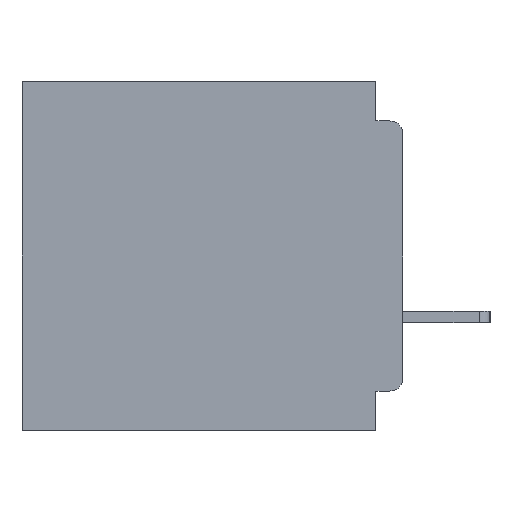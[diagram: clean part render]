
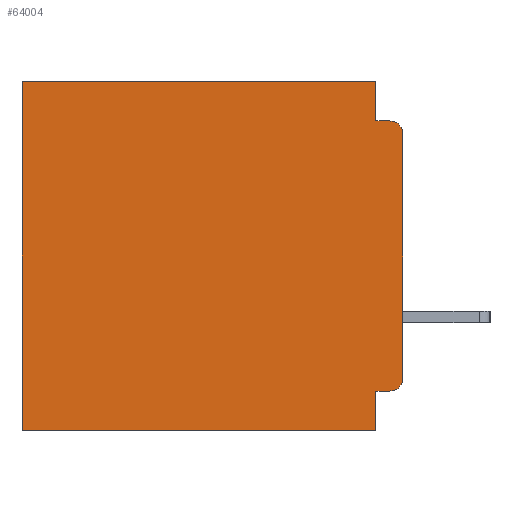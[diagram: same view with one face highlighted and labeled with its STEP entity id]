
A CAD part, left-side view. The second image highlights one B-rep face of the part: STEP entity #64004.
In plain terms, the highlighted planar face has unit normal (-1, 0, 0).
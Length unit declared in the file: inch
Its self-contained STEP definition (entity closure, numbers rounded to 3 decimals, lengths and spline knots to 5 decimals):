
#859 = CARTESIAN_POINT ( 'NONE',  ( 0.3, 0., -0.045 ) ) ;
#1046 = DIRECTION ( 'NONE',  ( 0., 0., -1. ) ) ;
#2041 = VERTEX_POINT ( 'NONE', #41027 ) ;
#2657 = VECTOR ( 'NONE', #32019, 39.37008 ) ;
#2817 = CIRCLE ( 'NONE', #4854, 0.015 ) ;
#3303 = VECTOR ( 'NONE', #16511, 39.37008 ) ;
#4626 = EDGE_LOOP ( 'NONE', ( #4662, #31064, #33483, #18555, #24308, #18602, #51033, #5411, #11930, #7686 ) ) ;
#4662 = ORIENTED_EDGE ( 'NONE', *, *, #42477, .F. ) ;
#4854 = AXIS2_PLACEMENT_3D ( 'NONE', #28053, #64151, #33227 ) ;
#5411 = ORIENTED_EDGE ( 'NONE', *, *, #32734, .F. ) ;
#6236 = CARTESIAN_POINT ( 'NONE',  ( 0.3, 0.437, -0.4 ) ) ;
#6506 = VECTOR ( 'NONE', #57713, 39.37008 ) ;
#6754 = CARTESIAN_POINT ( 'NONE',  ( 0.3, 0., -0.4 ) ) ;
#7686 = ORIENTED_EDGE ( 'NONE', *, *, #48527, .T. ) ;
#8101 = CARTESIAN_POINT ( 'NONE',  ( 0.3, 0., -0.06 ) ) ;
#9008 = EDGE_CURVE ( 'NONE', #2041, #52479, #17122, .T. ) ;
#9335 = CARTESIAN_POINT ( 'NONE',  ( 0.3, 0.031, 0. ) ) ;
#11239 = VECTOR ( 'NONE', #45523, 39.37008 ) ;
#11930 = ORIENTED_EDGE ( 'NONE', *, *, #64659, .F. ) ;
#12220 = DIRECTION ( 'NONE',  ( 0., 0., -1. ) ) ;
#13569 = DIRECTION ( 'NONE',  ( 0., 1., 0. ) ) ;
#13674 = CARTESIAN_POINT ( 'NONE',  ( 0.3, 0., -0.355 ) ) ;
#15152 = VECTOR ( 'NONE', #1046, 39.37008 ) ;
#15683 = VERTEX_POINT ( 'NONE', #22518 ) ;
#16511 = DIRECTION ( 'NONE',  ( 0., -1., 0. ) ) ;
#17122 = LINE ( 'NONE', #859, #3303 ) ;
#18555 = ORIENTED_EDGE ( 'NONE', *, *, #24389, .F. ) ;
#18602 = ORIENTED_EDGE ( 'NONE', *, *, #38197, .T. ) ;
#20509 = CARTESIAN_POINT ( 'NONE',  ( 0.3, 0.031, -0.355 ) ) ;
#20972 = CARTESIAN_POINT ( 'NONE',  ( 0.3, 0.015, -0.045 ) ) ;
#22061 = VERTEX_POINT ( 'NONE', #31079 ) ;
#22383 = VECTOR ( 'NONE', #13569, 39.37008 ) ;
#22518 = CARTESIAN_POINT ( 'NONE',  ( 0.3, 0.437, 0. ) ) ;
#24308 = ORIENTED_EDGE ( 'NONE', *, *, #30581, .T. ) ;
#24389 = EDGE_CURVE ( 'NONE', #38614, #2041, #47696, .T. ) ;
#24616 = VERTEX_POINT ( 'NONE', #31882 ) ;
#26933 = CARTESIAN_POINT ( 'NONE',  ( 0.3, 0.015, -0.34 ) ) ;
#27977 = DIRECTION ( 'NONE',  ( 0., 1., 0. ) ) ;
#28053 = CARTESIAN_POINT ( 'NONE',  ( 0.3, 0.015, -0.06 ) ) ;
#28451 = LINE ( 'NONE', #38400, #54408 ) ;
#28917 = LINE ( 'NONE', #6236, #15152 ) ;
#28929 = CARTESIAN_POINT ( 'NONE',  ( 0.3, 0., 0. ) ) ;
#30581 = EDGE_CURVE ( 'NONE', #38614, #15683, #49965, .T. ) ;
#31003 = VECTOR ( 'NONE', #39440, 39.37008 ) ;
#31064 = ORIENTED_EDGE ( 'NONE', *, *, #57271, .T. ) ;
#31079 = CARTESIAN_POINT ( 'NONE',  ( 0.3, 0.437, -0.4 ) ) ;
#31502 = VERTEX_POINT ( 'NONE', #37202 ) ;
#31882 = CARTESIAN_POINT ( 'NONE',  ( 0.3, 0.015, -0.355 ) ) ;
#32019 = DIRECTION ( 'NONE',  ( 0., 0., -1. ) ) ;
#32091 = DIRECTION ( 'NONE',  ( 0., 0., -1. ) ) ;
#32594 = LINE ( 'NONE', #13674, #31003 ) ;
#32734 = EDGE_CURVE ( 'NONE', #58212, #51086, #43962, .T. ) ;
#32753 = PLANE ( 'NONE',  #37023 ) ;
#33227 = DIRECTION ( 'NONE',  ( 0., 0., -1. ) ) ;
#33483 = ORIENTED_EDGE ( 'NONE', *, *, #9008, .F. ) ;
#34300 = EDGE_CURVE ( 'NONE', #51086, #22061, #28451, .T. ) ;
#34443 = CARTESIAN_POINT ( 'NONE',  ( 0.3, 0.031, -0.4 ) ) ;
#37023 = AXIS2_PLACEMENT_3D ( 'NONE', #6754, #43184, #12220 ) ;
#37202 = CARTESIAN_POINT ( 'NONE',  ( 0.3, 0., -0.34 ) ) ;
#38197 = EDGE_CURVE ( 'NONE', #15683, #22061, #28917, .T. ) ;
#38400 = CARTESIAN_POINT ( 'NONE',  ( 0.3, 0., -0.4 ) ) ;
#38614 = VERTEX_POINT ( 'NONE', #46744 ) ;
#39440 = DIRECTION ( 'NONE',  ( 0., 1., 0. ) ) ;
#40328 = CIRCLE ( 'NONE', #49655, 0.015 ) ;
#41027 = CARTESIAN_POINT ( 'NONE',  ( 0.3, 0.031, -0.045 ) ) ;
#42477 = EDGE_CURVE ( 'NONE', #62409, #31502, #59933, .T. ) ;
#43184 = DIRECTION ( 'NONE',  ( 1., 0., 0. ) ) ;
#43962 = LINE ( 'NONE', #47697, #2657 ) ;
#45523 = DIRECTION ( 'NONE',  ( 0., 0., -1. ) ) ;
#46744 = CARTESIAN_POINT ( 'NONE',  ( 0.3, 0.031, 0. ) ) ;
#47696 = LINE ( 'NONE', #9335, #11239 ) ;
#47697 = CARTESIAN_POINT ( 'NONE',  ( 0.3, 0.031, -0.4 ) ) ;
#48527 = EDGE_CURVE ( 'NONE', #24616, #31502, #40328, .T. ) ;
#49655 = AXIS2_PLACEMENT_3D ( 'NONE', #26933, #63038, #32091 ) ;
#49965 = LINE ( 'NONE', #28929, #22383 ) ;
#51033 = ORIENTED_EDGE ( 'NONE', *, *, #34300, .F. ) ;
#51086 = VERTEX_POINT ( 'NONE', #34443 ) ;
#52479 = VERTEX_POINT ( 'NONE', #20972 ) ;
#52559 = CARTESIAN_POINT ( 'NONE',  ( 0.3, 0., -0.4 ) ) ;
#54408 = VECTOR ( 'NONE', #27977, 39.37008 ) ;
#57271 = EDGE_CURVE ( 'NONE', #62409, #52479, #2817, .T. ) ;
#57713 = DIRECTION ( 'NONE',  ( 0., 0., -1. ) ) ;
#58212 = VERTEX_POINT ( 'NONE', #20509 ) ;
#59933 = LINE ( 'NONE', #52559, #6506 ) ;
#61007 = FACE_OUTER_BOUND ( 'NONE', #4626, .T. ) ;
#62409 = VERTEX_POINT ( 'NONE', #8101 ) ;
#63038 = DIRECTION ( 'NONE',  ( -1., 0., 0. ) ) ;
#64004 = ADVANCED_FACE ( 'NONE', ( #61007 ), #32753, .F. ) ;
#64151 = DIRECTION ( 'NONE',  ( -1., 0., 0. ) ) ;
#64659 = EDGE_CURVE ( 'NONE', #24616, #58212, #32594, .T. ) ;
